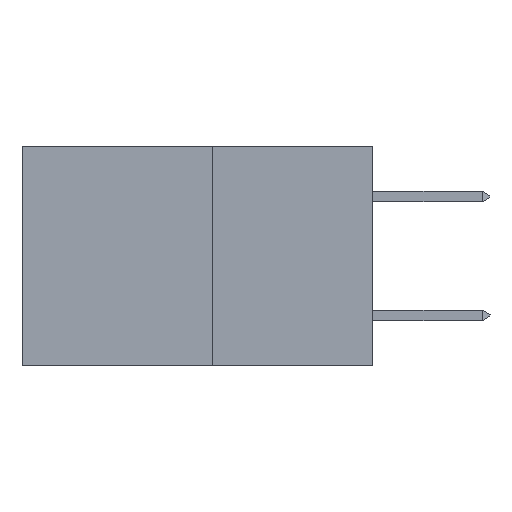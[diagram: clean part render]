
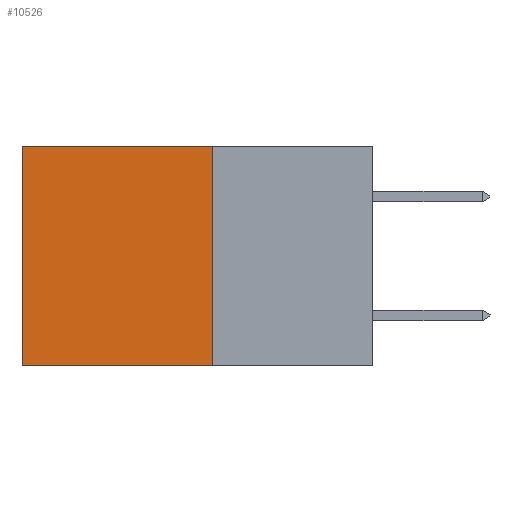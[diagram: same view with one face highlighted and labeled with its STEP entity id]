
A CAD part, left-side view. The second image highlights one B-rep face of the part: STEP entity #10526.
In plain terms, the highlighted planar face has unit normal (-1, 0, 0).
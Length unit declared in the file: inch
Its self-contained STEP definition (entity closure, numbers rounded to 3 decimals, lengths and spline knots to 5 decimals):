
#228 = LINE ( 'NONE', #6553, #8998 ) ;
#434 = VERTEX_POINT ( 'NONE', #7055 ) ;
#1429 = VECTOR ( 'NONE', #9288, 39.37008 ) ;
#1678 = LINE ( 'NONE', #12902, #13075 ) ;
#1995 = DIRECTION ( 'NONE',  ( 1., 0., 0. ) ) ;
#2620 = VERTEX_POINT ( 'NONE', #5898 ) ;
#2953 = AXIS2_PLACEMENT_3D ( 'NONE', #8663, #1995, #9769 ) ;
#4002 = ORIENTED_EDGE ( 'NONE', *, *, #8725, .F. ) ;
#4022 = EDGE_CURVE ( 'NONE', #11775, #434, #1678, .T. ) ;
#4585 = LINE ( 'NONE', #9343, #1429 ) ;
#4832 = CARTESIAN_POINT ( 'NONE',  ( 0.277, 0.27, -0.37 ) ) ;
#4872 = DIRECTION ( 'NONE',  ( 0., 1., 0. ) ) ;
#5628 = EDGE_CURVE ( 'NONE', #2620, #11775, #4585, .T. ) ;
#5898 = CARTESIAN_POINT ( 'NONE',  ( 0.277, 0.27, 0. ) ) ;
#6553 = CARTESIAN_POINT ( 'NONE',  ( 0.277, 0.27, -0.37 ) ) ;
#6570 = ORIENTED_EDGE ( 'NONE', *, *, #4022, .T. ) ;
#6650 = EDGE_CURVE ( 'NONE', #6832, #434, #14183, .T. ) ;
#6832 = VERTEX_POINT ( 'NONE', #14215 ) ;
#6907 = ORIENTED_EDGE ( 'NONE', *, *, #5628, .T. ) ;
#7055 = CARTESIAN_POINT ( 'NONE',  ( 0.277, 0.59, -0.37 ) ) ;
#7637 = DIRECTION ( 'NONE',  ( 0., 0., -1. ) ) ;
#8278 = VECTOR ( 'NONE', #4872, 39.37008 ) ;
#8663 = CARTESIAN_POINT ( 'NONE',  ( 0.277, 0.27, -0.37 ) ) ;
#8725 = EDGE_CURVE ( 'NONE', #2620, #6832, #228, .T. ) ;
#8962 = CARTESIAN_POINT ( 'NONE',  ( 0.277, 0.59, 0. ) ) ;
#8998 = VECTOR ( 'NONE', #7637, 39.37008 ) ;
#9288 = DIRECTION ( 'NONE',  ( 0., 1., 0. ) ) ;
#9343 = CARTESIAN_POINT ( 'NONE',  ( 0.277, 0.27, 0. ) ) ;
#9447 = ORIENTED_EDGE ( 'NONE', *, *, #6650, .F. ) ;
#9769 = DIRECTION ( 'NONE',  ( 0., 0., -1. ) ) ;
#10526 = ADVANCED_FACE ( 'NONE', ( #12064 ), #11969, .F. ) ;
#11775 = VERTEX_POINT ( 'NONE', #8962 ) ;
#11969 = PLANE ( 'NONE',  #2953 ) ;
#12064 = FACE_OUTER_BOUND ( 'NONE', #13175, .T. ) ;
#12727 = DIRECTION ( 'NONE',  ( 0., 0., -1. ) ) ;
#12902 = CARTESIAN_POINT ( 'NONE',  ( 0.277, 0.59, -0.37 ) ) ;
#13075 = VECTOR ( 'NONE', #12727, 39.37008 ) ;
#13175 = EDGE_LOOP ( 'NONE', ( #6570, #9447, #4002, #6907 ) ) ;
#14183 = LINE ( 'NONE', #4832, #8278 ) ;
#14215 = CARTESIAN_POINT ( 'NONE',  ( 0.277, 0.27, -0.37 ) ) ;
